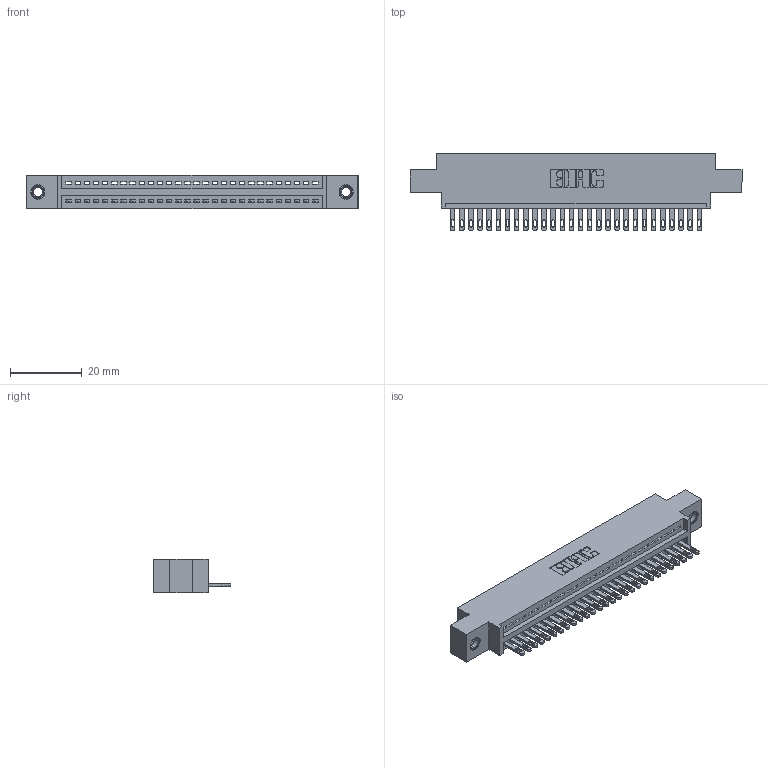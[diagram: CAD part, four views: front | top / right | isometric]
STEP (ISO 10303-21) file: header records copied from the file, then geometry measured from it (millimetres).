
FILE_DESCRIPTION (( 'STEP AP203' ), '1' );
FILE_NAME ('345-028-500-607.STEP', '2018-08-22T07:34:59', ( '' ), ( '' ), 'SwSTEP 2.0', 'SolidWorks 2016', '' );
FILE_SCHEMA (( 'CONFIG_CONTROL_DESIGN' ));
Length unit declared in the file: inch
Products named in the file (4): 345-292-001_345-293-100; 345-250-001_345-250-005-103; 345-028-500-607; 345 Part_0.170 Offset - 0.156 Dia-TI
Assembly tree (31 placements, depth 2):
  345-028-500-607
    345 Part_0.170 Offset - 0.156 Dia-TI
    345-292-001_345-293-100  x28
    345-250-001_345-250-005-103  x2
Bounding box: 92.33 x 21.51 x 9.4 mm (x, y, z)
Volume: 8545.3 mm3; surface area: 11387.6 mm2
Topology: 31 solids, 31 shells, 1702 faces, 5193 edges, 3454 vertices
Faces by surface type: plane 1068, cylinder 618, cone 12, torus 4
Entity records: 24206 total; most frequent: CARTESIAN_POINT 4175, ORIENTED_EDGE 4130, DIRECTION 3695, EDGE_CURVE 2065, VECTOR 1797, LINE 1797, VERTEX_POINT 1372, AXIS2_PLACEMENT_3D 949
